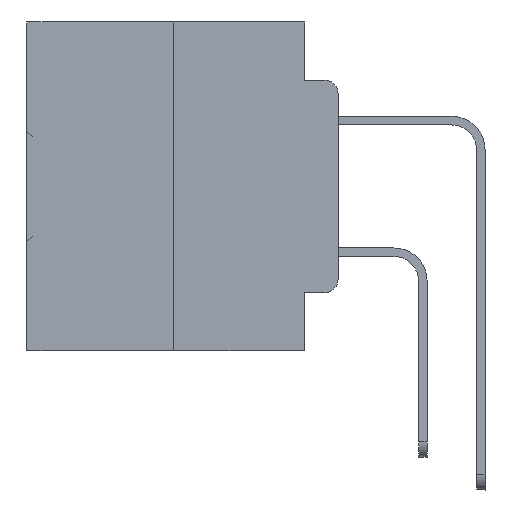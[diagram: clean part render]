
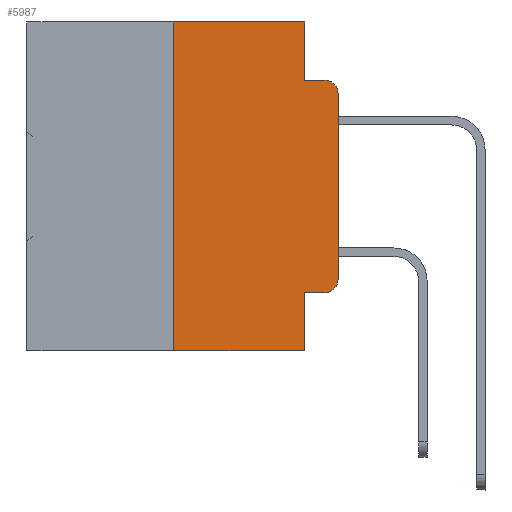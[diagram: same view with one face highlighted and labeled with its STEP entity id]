
A CAD part, left-side view. The second image highlights one B-rep face of the part: STEP entity #5987.
In plain terms, the highlighted planar face has unit normal (-1, 0, 0).
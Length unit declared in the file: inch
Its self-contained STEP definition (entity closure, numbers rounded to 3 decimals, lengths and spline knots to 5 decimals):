
#205 = ORIENTED_EDGE ( 'NONE', *, *, #8071, .F. ) ;
#1353 = CARTESIAN_POINT ( 'NONE',  ( 0., 0.051, -0.4115 ) ) ;
#1596 = EDGE_CURVE ( 'NONE', #9879, #25708, #9622, .T. ) ;
#1993 = ORIENTED_EDGE ( 'NONE', *, *, #33832, .F. ) ;
#2050 = VERTEX_POINT ( 'NONE', #5778 ) ;
#2305 = AXIS2_PLACEMENT_3D ( 'NONE', #6775, #15729, #18150 ) ;
#3178 = VERTEX_POINT ( 'NONE', #29919 ) ;
#3608 = AXIS2_PLACEMENT_3D ( 'NONE', #20590, #28824, #32369 ) ;
#3994 = FACE_OUTER_BOUND ( 'NONE', #34118, .T. ) ;
#5778 = CARTESIAN_POINT ( 'NONE',  ( 0., 0., -0.1085 ) ) ;
#5827 = CARTESIAN_POINT ( 'NONE',  ( 0., 0.051, 0. ) ) ;
#5987 = ADVANCED_FACE ( 'NONE', ( #3994 ), #15197, .F. ) ;
#6040 = EDGE_CURVE ( 'NONE', #14607, #26447, #26906, .T. ) ;
#6394 = VECTOR ( 'NONE', #31054, 39.37008 ) ;
#6650 = EDGE_CURVE ( 'NONE', #3178, #13322, #27753, .T. ) ;
#6775 = CARTESIAN_POINT ( 'NONE',  ( 0., 0.02, -0.1085 ) ) ;
#7579 = EDGE_CURVE ( 'NONE', #9879, #3178, #7741, .T. ) ;
#7741 = LINE ( 'NONE', #31085, #26642 ) ;
#8071 = EDGE_CURVE ( 'NONE', #20338, #17728, #36860, .T. ) ;
#8262 = CARTESIAN_POINT ( 'NONE',  ( 0., 0.051, -0.0885 ) ) ;
#8644 = LINE ( 'NONE', #10079, #27357 ) ;
#8943 = CARTESIAN_POINT ( 'NONE',  ( 0., 0.25, -0.5 ) ) ;
#9354 = CARTESIAN_POINT ( 'NONE',  ( 0., 0., -0.3915 ) ) ;
#9538 = EDGE_CURVE ( 'NONE', #25188, #2050, #8644, .T. ) ;
#9622 = LINE ( 'NONE', #20979, #31899 ) ;
#9879 = VERTEX_POINT ( 'NONE', #8943 ) ;
#9944 = ORIENTED_EDGE ( 'NONE', *, *, #33130, .F. ) ;
#9949 = DIRECTION ( 'NONE',  ( 0., 0., -1. ) ) ;
#10079 = CARTESIAN_POINT ( 'NONE',  ( 0., 0., 0. ) ) ;
#10265 = EDGE_CURVE ( 'NONE', #26447, #25188, #26210, .T. ) ;
#10583 = DIRECTION ( 'NONE',  ( 0., -1., 0. ) ) ;
#11087 = LINE ( 'NONE', #22444, #6394 ) ;
#11325 = CARTESIAN_POINT ( 'NONE',  ( 0., 0.473, 0. ) ) ;
#11619 = ORIENTED_EDGE ( 'NONE', *, *, #9538, .T. ) ;
#11788 = ORIENTED_EDGE ( 'NONE', *, *, #10265, .T. ) ;
#12078 = VECTOR ( 'NONE', #10583, 39.37008 ) ;
#12212 = DIRECTION ( 'NONE',  ( 1., 0., 0. ) ) ;
#12296 = CARTESIAN_POINT ( 'NONE',  ( 0., 0.051, -0.5 ) ) ;
#13012 = EDGE_CURVE ( 'NONE', #2050, #17728, #14830, .T. ) ;
#13317 = DIRECTION ( 'NONE',  ( 0., -1., 0. ) ) ;
#13322 = VERTEX_POINT ( 'NONE', #5827 ) ;
#14607 = VERTEX_POINT ( 'NONE', #24440 ) ;
#14830 = CIRCLE ( 'NONE', #2305, 0.02 ) ;
#14950 = CARTESIAN_POINT ( 'NONE',  ( 0., 0.051, 0. ) ) ;
#15197 = PLANE ( 'NONE',  #25533 ) ;
#15259 = ORIENTED_EDGE ( 'NONE', *, *, #6650, .F. ) ;
#15729 = DIRECTION ( 'NONE',  ( -1., 0., 0. ) ) ;
#15917 = VECTOR ( 'NONE', #20771, 39.37008 ) ;
#17728 = VERTEX_POINT ( 'NONE', #18624 ) ;
#18150 = DIRECTION ( 'NONE',  ( 0., 0., -1. ) ) ;
#18191 = DIRECTION ( 'NONE',  ( 0., -1., 0. ) ) ;
#18514 = CARTESIAN_POINT ( 'NONE',  ( 0., 0.473, 0. ) ) ;
#18624 = CARTESIAN_POINT ( 'NONE',  ( 0., 0.02, -0.0885 ) ) ;
#19704 = ORIENTED_EDGE ( 'NONE', *, *, #6040, .T. ) ;
#20338 = VERTEX_POINT ( 'NONE', #35994 ) ;
#20590 = CARTESIAN_POINT ( 'NONE',  ( 0., 0.02, -0.3915 ) ) ;
#20771 = DIRECTION ( 'NONE',  ( 0., -1., 0. ) ) ;
#20979 = CARTESIAN_POINT ( 'NONE',  ( 0., 0.473, -0.5 ) ) ;
#21756 = ORIENTED_EDGE ( 'NONE', *, *, #1596, .T. ) ;
#22444 = CARTESIAN_POINT ( 'NONE',  ( 0., 0.051, 0. ) ) ;
#22834 = CARTESIAN_POINT ( 'NONE',  ( 0., 0.02, -0.4115 ) ) ;
#23691 = LINE ( 'NONE', #14950, #31475 ) ;
#23886 = DIRECTION ( 'NONE',  ( 0., 0., 1. ) ) ;
#24440 = CARTESIAN_POINT ( 'NONE',  ( 0., 0.051, -0.4115 ) ) ;
#24849 = ORIENTED_EDGE ( 'NONE', *, *, #7579, .F. ) ;
#25088 = DIRECTION ( 'NONE',  ( 0., 0., 1. ) ) ;
#25188 = VERTEX_POINT ( 'NONE', #9354 ) ;
#25533 = AXIS2_PLACEMENT_3D ( 'NONE', #18514, #12212, #9949 ) ;
#25708 = VERTEX_POINT ( 'NONE', #12296 ) ;
#25910 = ORIENTED_EDGE ( 'NONE', *, *, #13012, .T. ) ;
#26210 = CIRCLE ( 'NONE', #3608, 0.02 ) ;
#26302 = DIRECTION ( 'NONE',  ( 0., 0., -1. ) ) ;
#26447 = VERTEX_POINT ( 'NONE', #22834 ) ;
#26642 = VECTOR ( 'NONE', #25088, 39.37008 ) ;
#26906 = LINE ( 'NONE', #1353, #15917 ) ;
#27254 = VECTOR ( 'NONE', #13317, 39.37008 ) ;
#27357 = VECTOR ( 'NONE', #23886, 39.37008 ) ;
#27753 = LINE ( 'NONE', #11325, #12078 ) ;
#28824 = DIRECTION ( 'NONE',  ( -1., 0., 0. ) ) ;
#29919 = CARTESIAN_POINT ( 'NONE',  ( 0., 0.25, 0. ) ) ;
#31054 = DIRECTION ( 'NONE',  ( 0., 0., -1. ) ) ;
#31085 = CARTESIAN_POINT ( 'NONE',  ( 0., 0.25, 0. ) ) ;
#31475 = VECTOR ( 'NONE', #26302, 39.37008 ) ;
#31899 = VECTOR ( 'NONE', #18191, 39.37008 ) ;
#32369 = DIRECTION ( 'NONE',  ( 0., 0., -1. ) ) ;
#33130 = EDGE_CURVE ( 'NONE', #13322, #20338, #11087, .T. ) ;
#33832 = EDGE_CURVE ( 'NONE', #14607, #25708, #23691, .T. ) ;
#34118 = EDGE_LOOP ( 'NONE', ( #11619, #25910, #205, #9944, #15259, #24849, #21756, #1993, #19704, #11788 ) ) ;
#35994 = CARTESIAN_POINT ( 'NONE',  ( 0., 0.051, -0.0885 ) ) ;
#36860 = LINE ( 'NONE', #8262, #27254 ) ;
